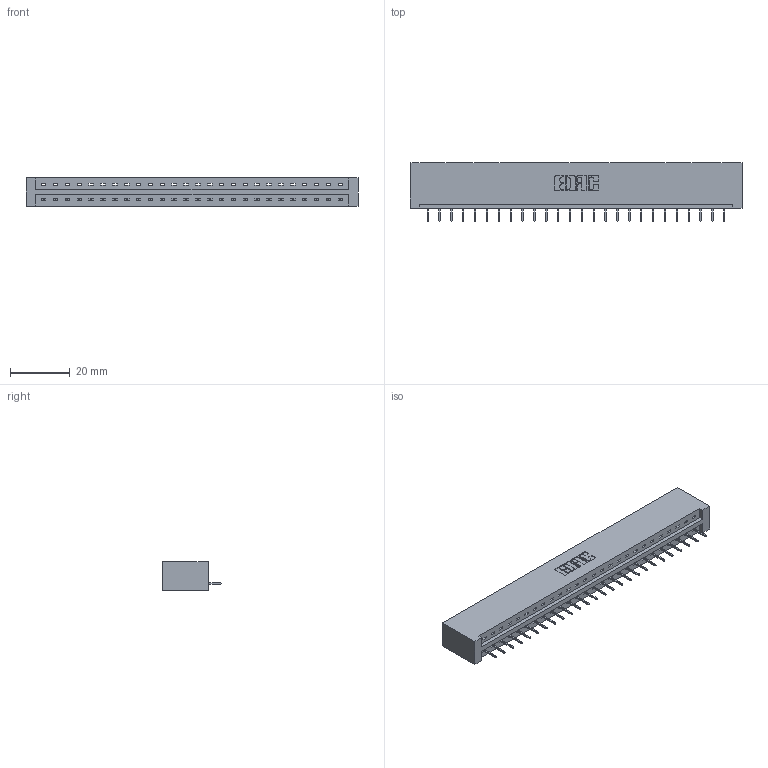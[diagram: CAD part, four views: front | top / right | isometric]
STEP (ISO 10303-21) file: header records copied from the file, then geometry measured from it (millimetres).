
FILE_DESCRIPTION (( 'STEP AP203' ), '1' );
FILE_NAME ('387-026-524-101.STEP', '2018-09-16T00:37:16', ( '' ), ( '' ), 'SwSTEP 2.0', 'SolidWorks 2016', '' );
FILE_SCHEMA (( 'CONFIG_CONTROL_DESIGN' ));
Length unit declared in the file: inch
Products named in the file (3): 337 Part_No Mounting Lugs; 345-292-001_345-293-124; 387-026-524-101
Assembly tree (27 placements, depth 2):
  387-026-524-101
    337 Part_No Mounting Lugs
    345-292-001_345-293-124  x26
Bounding box: 110.9 x 19.69 x 9.4 mm (x, y, z)
Volume: 11961.6 mm3; surface area: 11892 mm2
Topology: 27 solids, 27 shells, 1822 faces, 5279 edges, 3414 vertices
Faces by surface type: plane 1418, cylinder 404
Entity records: 21193 total; most frequent: CARTESIAN_POINT 3696, ORIENTED_EDGE 3658, DIRECTION 3137, EDGE_CURVE 1829, VECTOR 1713, LINE 1713, VERTEX_POINT 1214, AXIS2_PLACEMENT_3D 712
